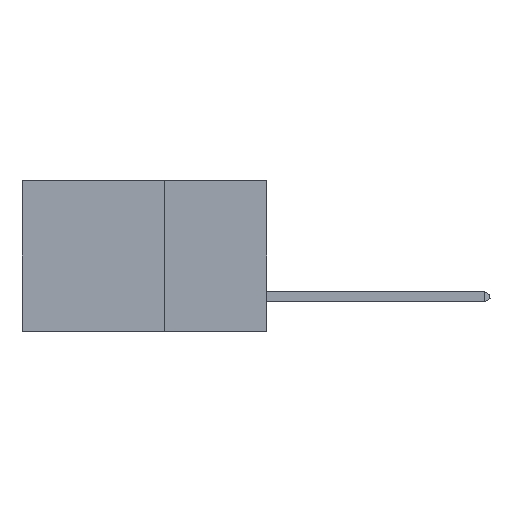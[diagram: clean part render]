
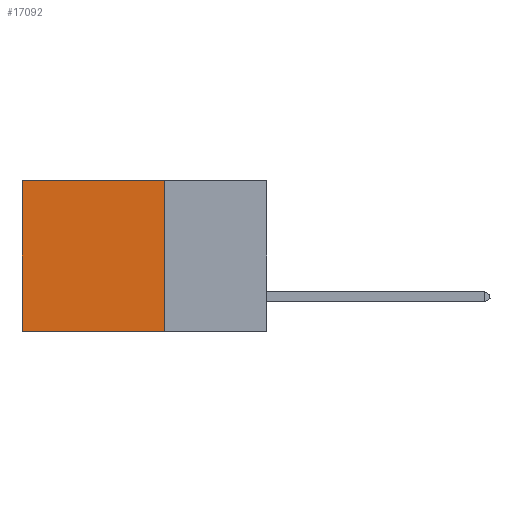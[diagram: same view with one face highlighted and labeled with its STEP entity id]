
A CAD part, left-side view. The second image highlights one B-rep face of the part: STEP entity #17092.
In plain terms, the highlighted planar face has unit normal (-1, 0, 0).
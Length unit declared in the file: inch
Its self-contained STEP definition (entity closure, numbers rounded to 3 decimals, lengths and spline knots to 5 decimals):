
#1480 = CARTESIAN_POINT ( 'NONE',  ( 0.2875, 0.6, 0. ) ) ;
#2605 = DIRECTION ( 'NONE',  ( 0., 0., -1. ) ) ;
#3630 = LINE ( 'NONE', #1480, #24155 ) ;
#3994 = LINE ( 'NONE', #19588, #19871 ) ;
#4354 = VERTEX_POINT ( 'NONE', #21451 ) ;
#5437 = CARTESIAN_POINT ( 'NONE',  ( 0.2875, 0.6, -0.37 ) ) ;
#5908 = CARTESIAN_POINT ( 'NONE',  ( 0.2875, 0.6, 0. ) ) ;
#8161 = EDGE_CURVE ( 'NONE', #4354, #19450, #16742, .T. ) ;
#11283 = CARTESIAN_POINT ( 'NONE',  ( 0.2875, 0.25, -0.37 ) ) ;
#12756 = DIRECTION ( 'NONE',  ( 1., 0., 0. ) ) ;
#13027 = FACE_OUTER_BOUND ( 'NONE', #16074, .T. ) ;
#13252 = VECTOR ( 'NONE', #29610, 39.37008 ) ;
#15067 = ORIENTED_EDGE ( 'NONE', *, *, #27961, .F. ) ;
#15138 = PLANE ( 'NONE',  #25049 ) ;
#16074 = EDGE_LOOP ( 'NONE', ( #19431, #15067, #19772, #24828 ) ) ;
#16645 = EDGE_CURVE ( 'NONE', #4354, #26596, #3994, .T. ) ;
#16742 = LINE ( 'NONE', #27182, #22862 ) ;
#17067 = DIRECTION ( 'NONE',  ( 0., 1., 0. ) ) ;
#17092 = ADVANCED_FACE ( 'NONE', ( #13027 ), #15138, .F. ) ;
#17108 = EDGE_CURVE ( 'NONE', #26596, #17558, #3630, .T. ) ;
#17528 = DIRECTION ( 'NONE',  ( 0., 0., -1. ) ) ;
#17558 = VERTEX_POINT ( 'NONE', #5437 ) ;
#19431 = ORIENTED_EDGE ( 'NONE', *, *, #17108, .T. ) ;
#19450 = VERTEX_POINT ( 'NONE', #24261 ) ;
#19588 = CARTESIAN_POINT ( 'NONE',  ( 0.2875, 0.25, 0. ) ) ;
#19772 = ORIENTED_EDGE ( 'NONE', *, *, #8161, .F. ) ;
#19871 = VECTOR ( 'NONE', #17067, 39.37008 ) ;
#21451 = CARTESIAN_POINT ( 'NONE',  ( 0.2875, 0.25, 0. ) ) ;
#21853 = LINE ( 'NONE', #11283, #13252 ) ;
#22862 = VECTOR ( 'NONE', #2605, 39.37008 ) ;
#24155 = VECTOR ( 'NONE', #17528, 39.37008 ) ;
#24261 = CARTESIAN_POINT ( 'NONE',  ( 0.2875, 0.25, -0.37 ) ) ;
#24287 = DIRECTION ( 'NONE',  ( 0., 0., -1. ) ) ;
#24393 = CARTESIAN_POINT ( 'NONE',  ( 0.2875, 0.25, 0. ) ) ;
#24828 = ORIENTED_EDGE ( 'NONE', *, *, #16645, .T. ) ;
#25049 = AXIS2_PLACEMENT_3D ( 'NONE', #24393, #12756, #24287 ) ;
#26596 = VERTEX_POINT ( 'NONE', #5908 ) ;
#27182 = CARTESIAN_POINT ( 'NONE',  ( 0.2875, 0.25, 0. ) ) ;
#27961 = EDGE_CURVE ( 'NONE', #19450, #17558, #21853, .T. ) ;
#29610 = DIRECTION ( 'NONE',  ( 0., 1., 0. ) ) ;
